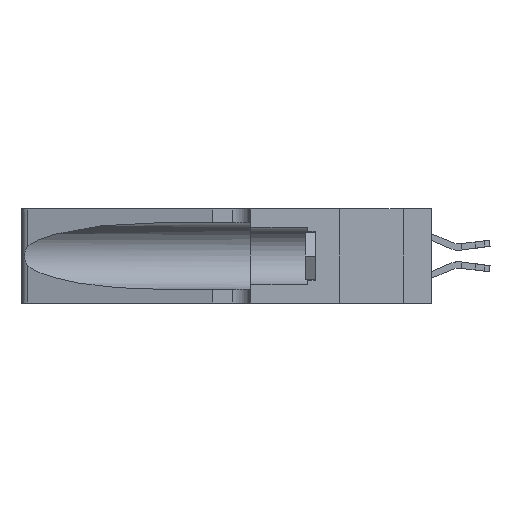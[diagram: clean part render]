
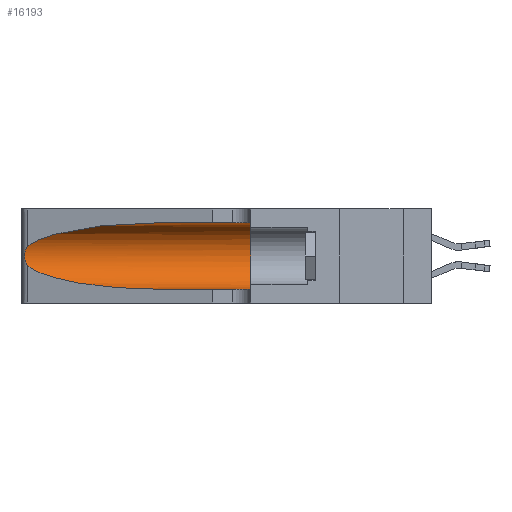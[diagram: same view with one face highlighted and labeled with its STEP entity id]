
A CAD part, left-side view. The second image highlights one B-rep face of the part: STEP entity #16193.
In plain terms, the highlighted cylindrical face has radius 3.308 mm (diameter 6.617 mm), a partial arc.
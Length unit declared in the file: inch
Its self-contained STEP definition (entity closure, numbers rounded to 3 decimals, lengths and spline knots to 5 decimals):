
#129 = CARTESIAN_POINT ( 'NONE',  ( 0.1305, 1.61858, 0.185 ) ) ;
#206 = ORIENTED_EDGE ( 'NONE', *, *, #13791, .F. ) ;
#2089 = CARTESIAN_POINT ( 'NONE',  ( 0.25487, 1.22718, 0.22369 ) ) ;
#2191 = CARTESIAN_POINT ( 'NONE',  ( 0.26075, 1.23896, 0.178 ) ) ;
#2201 =( BOUNDED_CURVE ( )  B_SPLINE_CURVE ( 3, ( #18762, #25732, #21139, #7164 ),
 .UNSPECIFIED., .F., .F. ) 
 B_SPLINE_CURVE_WITH_KNOTS ( ( 4, 4 ),
 ( 3.44316, 4.71239 ),
 .UNSPECIFIED. ) 
 CURVE ( )  GEOMETRIC_REPRESENTATION_ITEM ( )  RATIONAL_B_SPLINE_CURVE ( ( 1., 0.87, 0.87, 1. ) ) 
 REPRESENTATION_ITEM ( '' )  );
#3307 = VERTEX_POINT ( 'NONE', #8617 ) ;
#3764 = CARTESIAN_POINT ( 'NONE',  ( 0.1305, 1.61858, 0.31525 ) ) ;
#4248 = CARTESIAN_POINT ( 'NONE',  ( 0.25487, 1.22718, 0.22369 ) ) ;
#4592 = CARTESIAN_POINT ( 'NONE',  ( 0.25856, 1.23593, 0.16098 ) ) ;
#4771 = EDGE_CURVE ( 'NONE', #20438, #29687, #16404, .T. ) ;
#5557 = ORIENTED_EDGE ( 'NONE', *, *, #11417, .F. ) ;
#6353 = CARTESIAN_POINT ( 'NONE',  ( 0.25487, 1.22718, 0.14631 ) ) ;
#6978 = CARTESIAN_POINT ( 'NONE',  ( 0.25639, 1.23186, 0.15144 ) ) ;
#7164 = CARTESIAN_POINT ( 'NONE',  ( 0.1305, 0.72297, 0.05475 ) ) ;
#7540 = VERTEX_POINT ( 'NONE', #15907 ) ;
#8127 = CARTESIAN_POINT ( 'NONE',  ( 0.1305, 0.72297, 0.31525 ) ) ;
#8163 = CARTESIAN_POINT ( 'NONE',  ( 0.1305, 0.72297, 0.05475 ) ) ;
#8560 = VECTOR ( 'NONE', #24811, 39.37008 ) ;
#8617 = CARTESIAN_POINT ( 'NONE',  ( 0.1305, 0.35, 0.31525 ) ) ;
#8902 = CARTESIAN_POINT ( 'NONE',  ( 0.18966, 0.96281, 0.31525 ) ) ;
#8970 =( BOUNDED_CURVE ( )  B_SPLINE_CURVE ( 3, ( #11212, #8902, #18211, #4248 ),
 .UNSPECIFIED., .F., .F. ) 
 B_SPLINE_CURVE_WITH_KNOTS ( ( 4, 4 ),
 ( 1.5708, 2.84003 ),
 .UNSPECIFIED. ) 
 CURVE ( )  GEOMETRIC_REPRESENTATION_ITEM ( )  RATIONAL_B_SPLINE_CURVE ( ( 1., 0.87, 0.87, 1. ) ) 
 REPRESENTATION_ITEM ( '' )  );
#9157 = CARTESIAN_POINT ( 'NONE',  ( 0.25555, 1.22994, 0.2215 ) ) ;
#9214 = CIRCLE ( 'NONE', #17925, 0.13025 ) ;
#9354 = CARTESIAN_POINT ( 'NONE',  ( 0.25487, 1.22718, 0.14631 ) ) ;
#9392 = ORIENTED_EDGE ( 'NONE', *, *, #20003, .T. ) ;
#11070 = DIRECTION ( 'NONE',  ( 0., 1., 0. ) ) ;
#11212 = CARTESIAN_POINT ( 'NONE',  ( 0.1305, 0.72297, 0.31525 ) ) ;
#11341 = CYLINDRICAL_SURFACE ( 'NONE', #26270, 0.13025 ) ;
#11417 = EDGE_CURVE ( 'NONE', #3307, #29687, #9214, .T. ) ;
#11558 = CARTESIAN_POINT ( 'NONE',  ( 0.25639, 1.23184, 0.21858 ) ) ;
#11931 = DIRECTION ( 'NONE',  ( 0., 0., -1. ) ) ;
#13791 = EDGE_CURVE ( 'NONE', #21106, #3307, #20942, .T. ) ;
#13878 = CARTESIAN_POINT ( 'NONE',  ( 0.25854, 1.2359, 0.20912 ) ) ;
#14819 = EDGE_LOOP ( 'NONE', ( #9392, #26132, #26989, #28919, #5557, #206 ) ) ;
#14834 = CARTESIAN_POINT ( 'NONE',  ( 0.1305, 0.35, 0.05475 ) ) ;
#15143 = VERTEX_POINT ( 'NONE', #6353 ) ;
#15907 = CARTESIAN_POINT ( 'NONE',  ( 0.25487, 1.22718, 0.22369 ) ) ;
#16193 = ADVANCED_FACE ( 'NONE', ( #18241 ), #11341, .F. ) ;
#16254 = CARTESIAN_POINT ( 'NONE',  ( 0.26075, 1.23896, 0.19203 ) ) ;
#16404 = LINE ( 'NONE', #30110, #28815 ) ;
#17925 = AXIS2_PLACEMENT_3D ( 'NONE', #25043, #11070, #27398 ) ;
#18211 = CARTESIAN_POINT ( 'NONE',  ( 0.2373, 1.15595, 0.28018 ) ) ;
#18241 = FACE_OUTER_BOUND ( 'NONE', #14819, .T. ) ;
#18577 = CARTESIAN_POINT ( 'NONE',  ( 0.26017, 1.23833, 0.17102 ) ) ;
#18762 = CARTESIAN_POINT ( 'NONE',  ( 0.25487, 1.22718, 0.14631 ) ) ;
#18960 = DIRECTION ( 'NONE',  ( 0., -1., 0. ) ) ;
#19493 = EDGE_CURVE ( 'NONE', #15143, #20438, #2201, .T. ) ;
#20003 = EDGE_CURVE ( 'NONE', #21106, #7540, #8970, .T. ) ;
#20438 = VERTEX_POINT ( 'NONE', #8163 ) ;
#20657 = DIRECTION ( 'NONE',  ( 0., -1., 0. ) ) ;
#20942 = LINE ( 'NONE', #3764, #8560 ) ;
#20962 = CARTESIAN_POINT ( 'NONE',  ( 0.25789, 1.23486, 0.15765 ) ) ;
#21106 = VERTEX_POINT ( 'NONE', #8127 ) ;
#21139 = CARTESIAN_POINT ( 'NONE',  ( 0.18966, 0.96281, 0.05475 ) ) ;
#23289 = CARTESIAN_POINT ( 'NONE',  ( 0.25555, 1.22993, 0.14849 ) ) ;
#24502 = EDGE_CURVE ( 'NONE', #7540, #15143, #24925, .T. ) ;
#24811 = DIRECTION ( 'NONE',  ( 0., -1., 0. ) ) ;
#24925 = B_SPLINE_CURVE_WITH_KNOTS ( 'NONE', 3,
 ( #2089, #9157, #11558, #27884, #13878, #30220, #16254, #2191, #18577, #4592, #20962, #6978, #23289, #9354 ),
 .UNSPECIFIED., .F., .F.,
 ( 4, 2, 2, 2, 2, 2, 4 ),
 ( 0., 0.00027, 0.00053, 0.00107, 0.0016, 0.00187, 0.00214 ),
 .UNSPECIFIED. ) ;
#25043 = CARTESIAN_POINT ( 'NONE',  ( 0.1305, 0.35, 0.185 ) ) ;
#25732 = CARTESIAN_POINT ( 'NONE',  ( 0.2373, 1.15595, 0.08982 ) ) ;
#26132 = ORIENTED_EDGE ( 'NONE', *, *, #24502, .T. ) ;
#26270 = AXIS2_PLACEMENT_3D ( 'NONE', #129, #18960, #11931 ) ;
#26989 = ORIENTED_EDGE ( 'NONE', *, *, #19493, .T. ) ;
#27398 = DIRECTION ( 'NONE',  ( 0., 0., 1. ) ) ;
#27884 = CARTESIAN_POINT ( 'NONE',  ( 0.25787, 1.23484, 0.2124 ) ) ;
#28815 = VECTOR ( 'NONE', #20657, 39.37008 ) ;
#28919 = ORIENTED_EDGE ( 'NONE', *, *, #4771, .T. ) ;
#29687 = VERTEX_POINT ( 'NONE', #14834 ) ;
#30110 = CARTESIAN_POINT ( 'NONE',  ( 0.1305, 1.61858, 0.05475 ) ) ;
#30220 = CARTESIAN_POINT ( 'NONE',  ( 0.26018, 1.23835, 0.19895 ) ) ;
